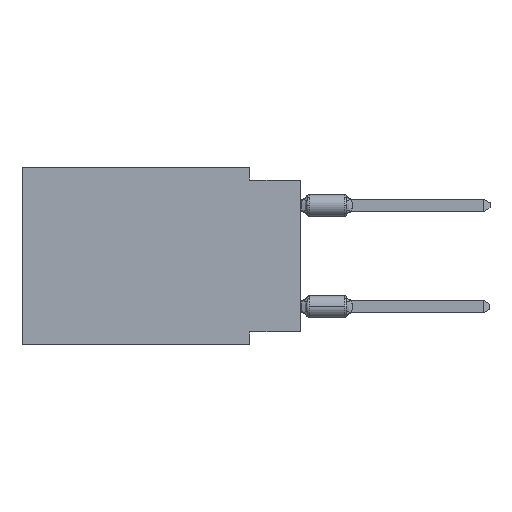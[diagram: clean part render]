
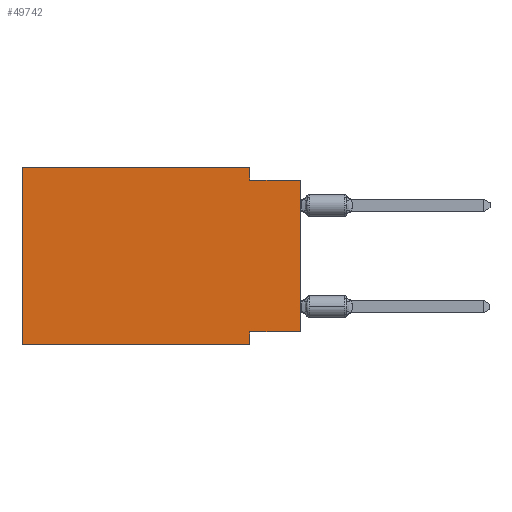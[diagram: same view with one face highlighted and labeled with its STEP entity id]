
A CAD part, left-side view. The second image highlights one B-rep face of the part: STEP entity #49742.
In plain terms, the highlighted planar face has unit normal (-1, 0, 0).
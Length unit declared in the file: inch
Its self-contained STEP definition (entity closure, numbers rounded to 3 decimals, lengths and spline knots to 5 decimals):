
#390 = ORIENTED_EDGE ( 'NONE', *, *, #71200, .F. ) ;
#928 = CARTESIAN_POINT ( 'NONE',  ( 0., 0.1, 0. ) ) ;
#956 = ORIENTED_EDGE ( 'NONE', *, *, #50947, .F. ) ;
#4014 = ORIENTED_EDGE ( 'NONE', *, *, #6712, .F. ) ;
#4593 = LINE ( 'NONE', #71273, #7754 ) ;
#4628 = CARTESIAN_POINT ( 'NONE',  ( 0., 0.1, -0.325 ) ) ;
#6710 = CARTESIAN_POINT ( 'NONE',  ( 0., 0., -0.325 ) ) ;
#6712 = EDGE_CURVE ( 'NONE', #12502, #71204, #44629, .T. ) ;
#7754 = VECTOR ( 'NONE', #60699, 39.37008 ) ;
#8777 = EDGE_CURVE ( 'NONE', #24361, #20770, #18394, .T. ) ;
#11458 = VECTOR ( 'NONE', #71035, 39.37008 ) ;
#11936 = VERTEX_POINT ( 'NONE', #54796 ) ;
#12208 = EDGE_CURVE ( 'NONE', #38871, #38099, #27644, .T. ) ;
#12502 = VERTEX_POINT ( 'NONE', #14811 ) ;
#14811 = CARTESIAN_POINT ( 'NONE',  ( 0., 0., -0.325 ) ) ;
#15100 = VECTOR ( 'NONE', #52891, 39.37008 ) ;
#15434 = CARTESIAN_POINT ( 'NONE',  ( 0., 0.55, 0. ) ) ;
#18394 = LINE ( 'NONE', #928, #55705 ) ;
#20262 = EDGE_CURVE ( 'NONE', #12502, #45264, #4593, .T. ) ;
#20770 = VERTEX_POINT ( 'NONE', #34339 ) ;
#22393 = VECTOR ( 'NONE', #65141, 39.37008 ) ;
#24295 = CARTESIAN_POINT ( 'NONE',  ( 0., 0.1, -0.35 ) ) ;
#24361 = VERTEX_POINT ( 'NONE', #38932 ) ;
#27644 = LINE ( 'NONE', #49858, #15100 ) ;
#28073 = EDGE_CURVE ( 'NONE', #20770, #45264, #61182, .T. ) ;
#32518 = ORIENTED_EDGE ( 'NONE', *, *, #28073, .F. ) ;
#34042 = DIRECTION ( 'NONE',  ( 0., 1., 0. ) ) ;
#34339 = CARTESIAN_POINT ( 'NONE',  ( 0., 0.1, -0.025 ) ) ;
#36022 = VECTOR ( 'NONE', #67297, 39.37008 ) ;
#36932 = PLANE ( 'NONE',  #65245 ) ;
#37662 = CARTESIAN_POINT ( 'NONE',  ( 0., 0.55, -0.35 ) ) ;
#37666 = DIRECTION ( 'NONE',  ( 1., 0., 0. ) ) ;
#37928 = ORIENTED_EDGE ( 'NONE', *, *, #12208, .T. ) ;
#38099 = VERTEX_POINT ( 'NONE', #24295 ) ;
#38871 = VERTEX_POINT ( 'NONE', #37662 ) ;
#38932 = CARTESIAN_POINT ( 'NONE',  ( 0., 0.1, 0. ) ) ;
#39893 = EDGE_CURVE ( 'NONE', #71204, #38099, #50526, .T. ) ;
#40923 = VECTOR ( 'NONE', #54440, 39.37008 ) ;
#42755 = CARTESIAN_POINT ( 'NONE',  ( 0., 0., -0.025 ) ) ;
#43611 = CARTESIAN_POINT ( 'NONE',  ( 0., 0.55, 0. ) ) ;
#43843 = ORIENTED_EDGE ( 'NONE', *, *, #20262, .T. ) ;
#43967 = LINE ( 'NONE', #43611, #22393 ) ;
#44629 = LINE ( 'NONE', #6710, #52076 ) ;
#45264 = VERTEX_POINT ( 'NONE', #42755 ) ;
#49717 = EDGE_LOOP ( 'NONE', ( #43843, #32518, #70739, #390, #956, #37928, #56078, #4014 ) ) ;
#49742 = ADVANCED_FACE ( 'NONE', ( #60258 ), #36932, .F. ) ;
#49858 = CARTESIAN_POINT ( 'NONE',  ( 0., 0.55, -0.35 ) ) ;
#50526 = LINE ( 'NONE', #56365, #36022 ) ;
#50947 = EDGE_CURVE ( 'NONE', #38871, #11936, #53716, .T. ) ;
#51911 = DIRECTION ( 'NONE',  ( 0., 0., -1. ) ) ;
#52076 = VECTOR ( 'NONE', #34042, 39.37008 ) ;
#52891 = DIRECTION ( 'NONE',  ( 0., -1., 0. ) ) ;
#53716 = LINE ( 'NONE', #54079, #40923 ) ;
#54079 = CARTESIAN_POINT ( 'NONE',  ( 0., 0.55, 0. ) ) ;
#54440 = DIRECTION ( 'NONE',  ( 0., 0., 1. ) ) ;
#54796 = CARTESIAN_POINT ( 'NONE',  ( 0., 0.55, 0. ) ) ;
#55705 = VECTOR ( 'NONE', #51911, 39.37008 ) ;
#56078 = ORIENTED_EDGE ( 'NONE', *, *, #39893, .F. ) ;
#56365 = CARTESIAN_POINT ( 'NONE',  ( 0., 0.1, -0.35 ) ) ;
#59898 = DIRECTION ( 'NONE',  ( 0., 0., -1. ) ) ;
#60258 = FACE_OUTER_BOUND ( 'NONE', #49717, .T. ) ;
#60699 = DIRECTION ( 'NONE',  ( 0., 0., 1. ) ) ;
#61182 = LINE ( 'NONE', #66656, #11458 ) ;
#65141 = DIRECTION ( 'NONE',  ( 0., -1., 0. ) ) ;
#65245 = AXIS2_PLACEMENT_3D ( 'NONE', #15434, #37666, #59898 ) ;
#66656 = CARTESIAN_POINT ( 'NONE',  ( 0., 0., -0.025 ) ) ;
#67297 = DIRECTION ( 'NONE',  ( 0., 0., -1. ) ) ;
#70739 = ORIENTED_EDGE ( 'NONE', *, *, #8777, .F. ) ;
#71035 = DIRECTION ( 'NONE',  ( 0., -1., 0. ) ) ;
#71200 = EDGE_CURVE ( 'NONE', #11936, #24361, #43967, .T. ) ;
#71204 = VERTEX_POINT ( 'NONE', #4628 ) ;
#71273 = CARTESIAN_POINT ( 'NONE',  ( 0., 0., 0. ) ) ;
